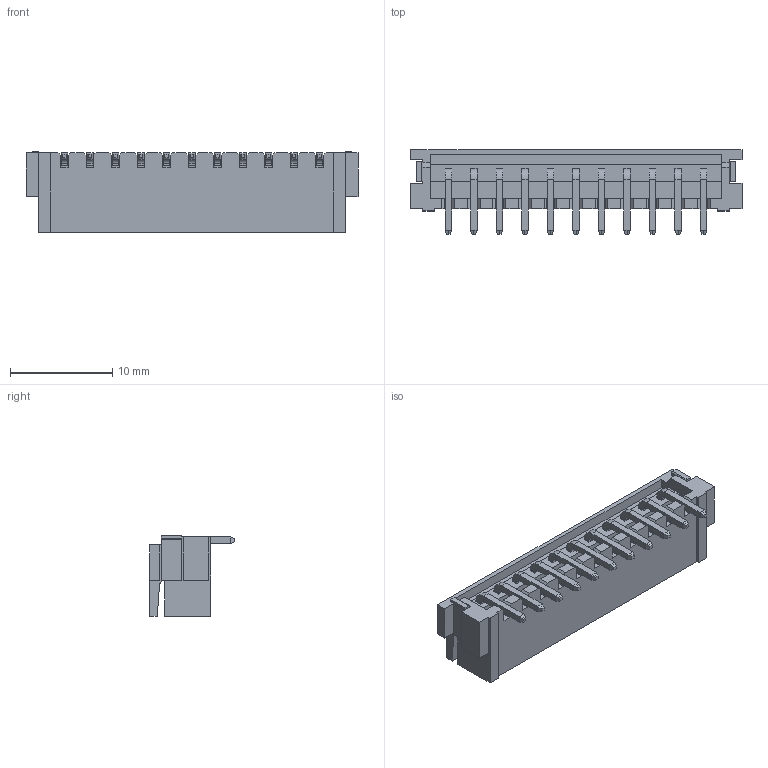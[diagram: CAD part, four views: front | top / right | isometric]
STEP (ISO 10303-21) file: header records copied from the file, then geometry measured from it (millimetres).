
FILE_DESCRIPTION (( 'STEP AP203' ), '1' );
FILE_NAME ('14K-511-418TAA1.STEP', '2024-02-22T14:32:01', ( '' ), ( '' ), 'SwSTEP 2.0', 'SolidWorks 2023', '' );
FILE_SCHEMA (( 'CONFIG_CONTROL_DESIGN' ));
Length unit declared in the file: millimetre
Products named in the file (3): 14K Series SMT Top Entry Insulator_511; 14K Series SMT Pin_Top Entry; 14K-511-418TAA1
Assembly tree (12 placements, depth 2):
  14K-511-418TAA1
    14K Series SMT Top Entry Insulator_511
    14K Series SMT Pin_Top Entry  x11
Bounding box: 32.5 x 8.3 x 7.9 mm (x, y, z)
Volume: 581.6 mm3; surface area: 1849 mm2
Topology: 12 solids, 12 shells, 566 faces, 1420 edges, 878 vertices
Faces by surface type: plane 516, cylinder 50
Entity records: 10987 total; most frequent: CARTESIAN_POINT 1865, ORIENTED_EDGE 1840, DIRECTION 1660, EDGE_CURVE 920, LINE 858, VECTOR 858, VERTEX_POINT 598, AXIS2_PLACEMENT_3D 401
